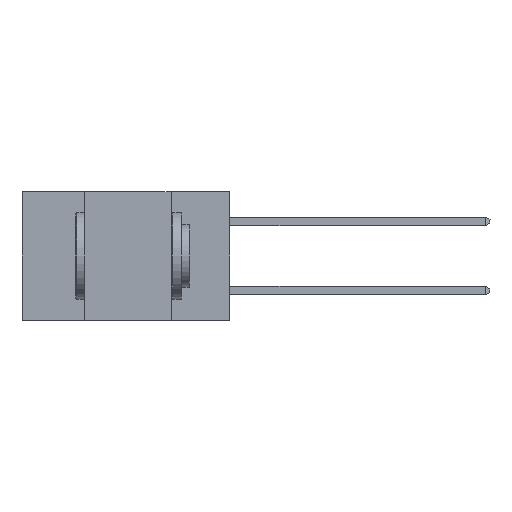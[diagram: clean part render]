
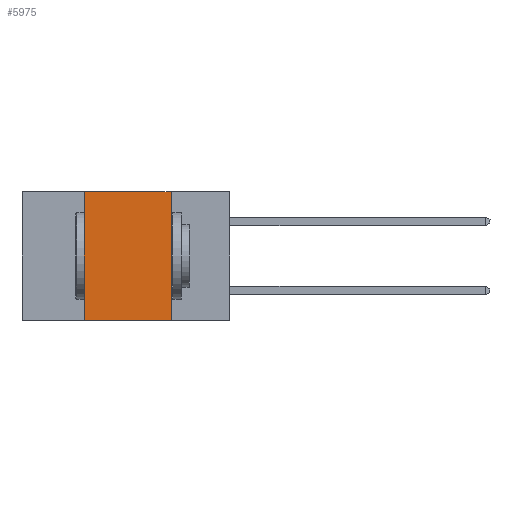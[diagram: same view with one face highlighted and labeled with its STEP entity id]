
A CAD part, left-side view. The second image highlights one B-rep face of the part: STEP entity #5975.
In plain terms, the highlighted planar face has unit normal (-1, 0, 0).
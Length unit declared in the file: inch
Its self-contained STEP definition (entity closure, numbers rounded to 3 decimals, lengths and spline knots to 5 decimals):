
#700 = LINE ( 'NONE', #10526, #5525 ) ;
#828 = LINE ( 'NONE', #1596, #1872 ) ;
#1093 = CARTESIAN_POINT ( 'NONE',  ( 0., 0.6, -0.37 ) ) ;
#1206 = FACE_OUTER_BOUND ( 'NONE', #4348, .T. ) ;
#1412 = EDGE_CURVE ( 'NONE', #10551, #5895, #828, .T. ) ;
#1596 = CARTESIAN_POINT ( 'NONE',  ( 0., 0.6, 0. ) ) ;
#1607 = CARTESIAN_POINT ( 'NONE',  ( 0., 0.42, -0.37 ) ) ;
#1872 = VECTOR ( 'NONE', #10605, 39.37008 ) ;
#2304 = ORIENTED_EDGE ( 'NONE', *, *, #10552, .F. ) ;
#2409 = CARTESIAN_POINT ( 'NONE',  ( 0., 0.42, 0. ) ) ;
#3168 = DIRECTION ( 'NONE',  ( 0., 0., 1. ) ) ;
#3529 = EDGE_CURVE ( 'NONE', #5895, #3750, #700, .T. ) ;
#3750 = VERTEX_POINT ( 'NONE', #6802 ) ;
#3984 = VECTOR ( 'NONE', #9348, 39.37008 ) ;
#4054 = AXIS2_PLACEMENT_3D ( 'NONE', #8696, #7845, #6246 ) ;
#4141 = EDGE_CURVE ( 'NONE', #8584, #3750, #7527, .T. ) ;
#4348 = EDGE_LOOP ( 'NONE', ( #9535, #4946, #2304, #9049 ) ) ;
#4413 = CARTESIAN_POINT ( 'NONE',  ( 0., 0.17, 0. ) ) ;
#4847 = LINE ( 'NONE', #1607, #7903 ) ;
#4946 = ORIENTED_EDGE ( 'NONE', *, *, #1412, .F. ) ;
#5525 = VECTOR ( 'NONE', #5626, 39.37008 ) ;
#5626 = DIRECTION ( 'NONE',  ( 0., 0., -1. ) ) ;
#5895 = VERTEX_POINT ( 'NONE', #4413 ) ;
#5975 = ADVANCED_FACE ( 'NONE', ( #1206 ), #7787, .F. ) ;
#6246 = DIRECTION ( 'NONE',  ( 0., 0., -1. ) ) ;
#6802 = CARTESIAN_POINT ( 'NONE',  ( 0., 0.17, -0.37 ) ) ;
#7527 = LINE ( 'NONE', #1093, #3984 ) ;
#7787 = PLANE ( 'NONE',  #4054 ) ;
#7845 = DIRECTION ( 'NONE',  ( 1., 0., 0. ) ) ;
#7903 = VECTOR ( 'NONE', #3168, 39.37008 ) ;
#8584 = VERTEX_POINT ( 'NONE', #10521 ) ;
#8696 = CARTESIAN_POINT ( 'NONE',  ( 0., 0.6, 0. ) ) ;
#9049 = ORIENTED_EDGE ( 'NONE', *, *, #4141, .T. ) ;
#9348 = DIRECTION ( 'NONE',  ( 0., -1., 0. ) ) ;
#9535 = ORIENTED_EDGE ( 'NONE', *, *, #3529, .F. ) ;
#10521 = CARTESIAN_POINT ( 'NONE',  ( 0., 0.42, -0.37 ) ) ;
#10526 = CARTESIAN_POINT ( 'NONE',  ( 0., 0.17, -0.37 ) ) ;
#10551 = VERTEX_POINT ( 'NONE', #2409 ) ;
#10552 = EDGE_CURVE ( 'NONE', #8584, #10551, #4847, .T. ) ;
#10605 = DIRECTION ( 'NONE',  ( 0., -1., 0. ) ) ;
